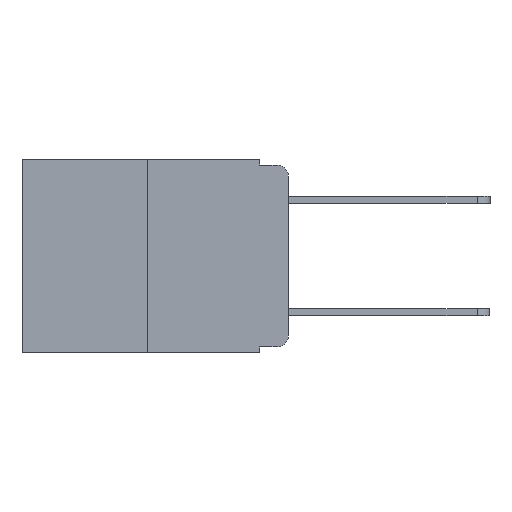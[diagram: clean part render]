
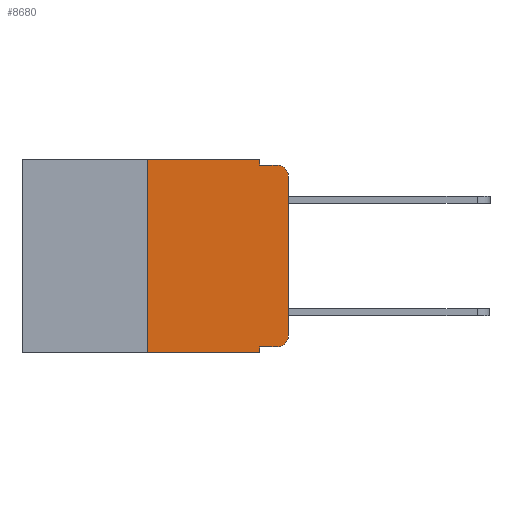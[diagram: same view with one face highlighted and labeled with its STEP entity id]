
A CAD part, left-side view. The second image highlights one B-rep face of the part: STEP entity #8680.
In plain terms, the highlighted planar face has unit normal (-1, 0, 0).
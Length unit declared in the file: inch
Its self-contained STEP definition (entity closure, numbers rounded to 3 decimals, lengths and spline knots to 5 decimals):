
#75 = EDGE_CURVE ( 'NONE', #9428, #4342, #5155, .T. ) ;
#217 = DIRECTION ( 'NONE',  ( 0., 0., -1. ) ) ;
#250 = ORIENTED_EDGE ( 'NONE', *, *, #1235, .F. ) ;
#382 = CARTESIAN_POINT ( 'NONE',  ( 0., 0.25, -0.343 ) ) ;
#405 = CARTESIAN_POINT ( 'NONE',  ( 0., 0.051, 0. ) ) ;
#607 = VERTEX_POINT ( 'NONE', #4770 ) ;
#749 = CARTESIAN_POINT ( 'NONE',  ( 0., 0.473, 0. ) ) ;
#916 = DIRECTION ( 'NONE',  ( 0., -1., 0. ) ) ;
#1110 = EDGE_CURVE ( 'NONE', #607, #9428, #4259, .T. ) ;
#1235 = EDGE_CURVE ( 'NONE', #2675, #6892, #7898, .T. ) ;
#1473 = VERTEX_POINT ( 'NONE', #3557 ) ;
#1736 = VECTOR ( 'NONE', #4807, 39.37008 ) ;
#2327 = DIRECTION ( 'NONE',  ( 0., 0., -1. ) ) ;
#2536 = EDGE_CURVE ( 'NONE', #1473, #2581, #2874, .T. ) ;
#2541 = CIRCLE ( 'NONE', #8203, 0.02 ) ;
#2581 = VERTEX_POINT ( 'NONE', #9072 ) ;
#2675 = VERTEX_POINT ( 'NONE', #11056 ) ;
#2748 = VECTOR ( 'NONE', #6022, 39.37008 ) ;
#2844 = EDGE_CURVE ( 'NONE', #2675, #6972, #9427, .T. ) ;
#2874 = LINE ( 'NONE', #8965, #7729 ) ;
#3013 = EDGE_CURVE ( 'NONE', #2581, #10459, #2541, .T. ) ;
#3118 = AXIS2_PLACEMENT_3D ( 'NONE', #4193, #10775, #5196 ) ;
#3220 = CARTESIAN_POINT ( 'NONE',  ( 0., 0.051, 0. ) ) ;
#3247 = LINE ( 'NONE', #10537, #3558 ) ;
#3557 = CARTESIAN_POINT ( 'NONE',  ( 0., 0., -0.313 ) ) ;
#3558 = VECTOR ( 'NONE', #916, 39.37008 ) ;
#3570 = ORIENTED_EDGE ( 'NONE', *, *, #2536, .T. ) ;
#3736 = VERTEX_POINT ( 'NONE', #382 ) ;
#3900 = ORIENTED_EDGE ( 'NONE', *, *, #10868, .T. ) ;
#4155 = LINE ( 'NONE', #9669, #10503 ) ;
#4193 = CARTESIAN_POINT ( 'NONE',  ( 0., 0.02, -0.313 ) ) ;
#4259 = LINE ( 'NONE', #749, #11430 ) ;
#4342 = VERTEX_POINT ( 'NONE', #8647 ) ;
#4770 = CARTESIAN_POINT ( 'NONE',  ( 0., 0.25, 0. ) ) ;
#4789 = ORIENTED_EDGE ( 'NONE', *, *, #75, .F. ) ;
#4807 = DIRECTION ( 'NONE',  ( 0., -1., 0. ) ) ;
#4944 = CARTESIAN_POINT ( 'NONE',  ( 0., 0.051, -0.333 ) ) ;
#4947 = VECTOR ( 'NONE', #8278, 39.37008 ) ;
#4956 = CARTESIAN_POINT ( 'NONE',  ( 0., 0.02, -0.01 ) ) ;
#5155 = LINE ( 'NONE', #405, #12242 ) ;
#5196 = DIRECTION ( 'NONE',  ( 0., 0., -1. ) ) ;
#5277 = ORIENTED_EDGE ( 'NONE', *, *, #10467, .F. ) ;
#5460 = CARTESIAN_POINT ( 'NONE',  ( 0., 0.051, -0.01 ) ) ;
#5719 = EDGE_LOOP ( 'NONE', ( #3570, #6489, #8230, #4789, #6816, #5277, #3900, #250, #9546, #7110 ) ) ;
#6001 = CIRCLE ( 'NONE', #3118, 0.02 ) ;
#6022 = DIRECTION ( 'NONE',  ( 0., 0., -1. ) ) ;
#6226 = DIRECTION ( 'NONE',  ( 1., 0., 0. ) ) ;
#6308 = FACE_OUTER_BOUND ( 'NONE', #5719, .T. ) ;
#6489 = ORIENTED_EDGE ( 'NONE', *, *, #3013, .T. ) ;
#6816 = ORIENTED_EDGE ( 'NONE', *, *, #1110, .F. ) ;
#6892 = VERTEX_POINT ( 'NONE', #11809 ) ;
#6972 = VERTEX_POINT ( 'NONE', #7238 ) ;
#7110 = ORIENTED_EDGE ( 'NONE', *, *, #11883, .T. ) ;
#7238 = CARTESIAN_POINT ( 'NONE',  ( 0., 0.02, -0.333 ) ) ;
#7405 = EDGE_CURVE ( 'NONE', #4342, #10459, #9938, .T. ) ;
#7547 = AXIS2_PLACEMENT_3D ( 'NONE', #8157, #6226, #217 ) ;
#7729 = VECTOR ( 'NONE', #8973, 39.37008 ) ;
#7898 = LINE ( 'NONE', #3220, #2748 ) ;
#8157 = CARTESIAN_POINT ( 'NONE',  ( 0., 0.473, 0. ) ) ;
#8203 = AXIS2_PLACEMENT_3D ( 'NONE', #12376, #12355, #12344 ) ;
#8230 = ORIENTED_EDGE ( 'NONE', *, *, #7405, .F. ) ;
#8278 = DIRECTION ( 'NONE',  ( 0., -1., 0. ) ) ;
#8293 = CARTESIAN_POINT ( 'NONE',  ( 0., 0.051, 0. ) ) ;
#8647 = CARTESIAN_POINT ( 'NONE',  ( 0., 0.051, -0.01 ) ) ;
#8680 = ADVANCED_FACE ( 'NONE', ( #6308 ), #11680, .F. ) ;
#8965 = CARTESIAN_POINT ( 'NONE',  ( 0., 0., 0. ) ) ;
#8973 = DIRECTION ( 'NONE',  ( 0., 0., 1. ) ) ;
#9072 = CARTESIAN_POINT ( 'NONE',  ( 0., 0., -0.03 ) ) ;
#9427 = LINE ( 'NONE', #4944, #1736 ) ;
#9428 = VERTEX_POINT ( 'NONE', #8293 ) ;
#9546 = ORIENTED_EDGE ( 'NONE', *, *, #2844, .T. ) ;
#9669 = CARTESIAN_POINT ( 'NONE',  ( 0., 0.25, 0. ) ) ;
#9938 = LINE ( 'NONE', #5460, #4947 ) ;
#10459 = VERTEX_POINT ( 'NONE', #4956 ) ;
#10467 = EDGE_CURVE ( 'NONE', #3736, #607, #4155, .T. ) ;
#10503 = VECTOR ( 'NONE', #12352, 39.37008 ) ;
#10537 = CARTESIAN_POINT ( 'NONE',  ( 0., 0.473, -0.343 ) ) ;
#10775 = DIRECTION ( 'NONE',  ( -1., 0., 0. ) ) ;
#10868 = EDGE_CURVE ( 'NONE', #3736, #6892, #3247, .T. ) ;
#11056 = CARTESIAN_POINT ( 'NONE',  ( 0., 0.051, -0.333 ) ) ;
#11430 = VECTOR ( 'NONE', #12017, 39.37008 ) ;
#11680 = PLANE ( 'NONE',  #7547 ) ;
#11809 = CARTESIAN_POINT ( 'NONE',  ( 0., 0.051, -0.343 ) ) ;
#11883 = EDGE_CURVE ( 'NONE', #6972, #1473, #6001, .T. ) ;
#12017 = DIRECTION ( 'NONE',  ( 0., -1., 0. ) ) ;
#12242 = VECTOR ( 'NONE', #2327, 39.37008 ) ;
#12344 = DIRECTION ( 'NONE',  ( 0., 0., -1. ) ) ;
#12352 = DIRECTION ( 'NONE',  ( 0., 0., 1. ) ) ;
#12355 = DIRECTION ( 'NONE',  ( -1., 0., 0. ) ) ;
#12376 = CARTESIAN_POINT ( 'NONE',  ( 0., 0.02, -0.03 ) ) ;
